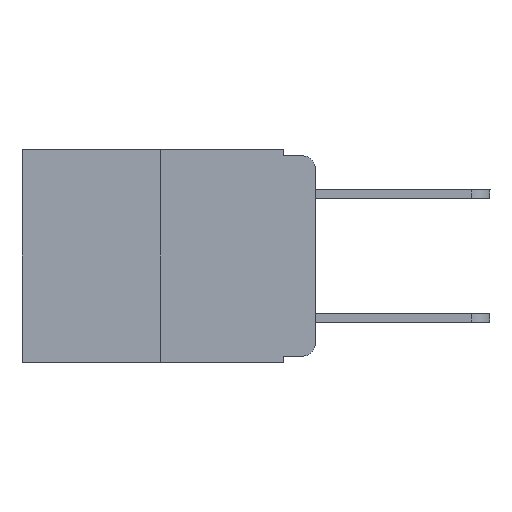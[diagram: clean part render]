
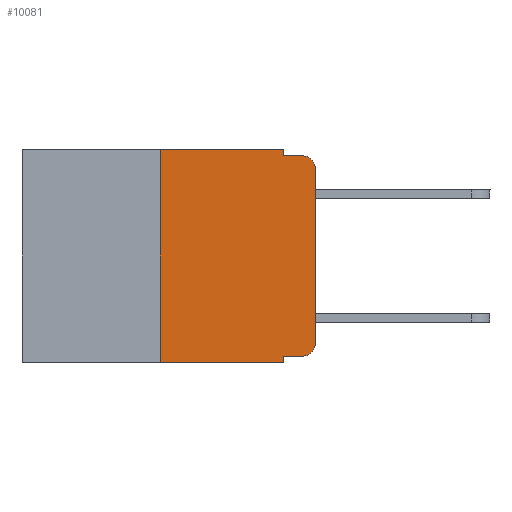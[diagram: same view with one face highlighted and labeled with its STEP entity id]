
A CAD part, left-side view. The second image highlights one B-rep face of the part: STEP entity #10081.
In plain terms, the highlighted planar face has unit normal (-1, 0, 0).
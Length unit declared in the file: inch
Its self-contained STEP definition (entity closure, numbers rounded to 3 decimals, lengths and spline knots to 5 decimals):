
#12 = LINE ( 'NONE', #4624, #12242 ) ;
#532 = LINE ( 'NONE', #13528, #14989 ) ;
#535 = CARTESIAN_POINT ( 'NONE',  ( 0., 0.473, 0. ) ) ;
#575 = LINE ( 'NONE', #5580, #6875 ) ;
#1215 = ORIENTED_EDGE ( 'NONE', *, *, #10044, .T. ) ;
#1301 = ORIENTED_EDGE ( 'NONE', *, *, #13924, .F. ) ;
#1306 = CARTESIAN_POINT ( 'NONE',  ( 0., 0.051, -0.333 ) ) ;
#1448 = VERTEX_POINT ( 'NONE', #2117 ) ;
#1495 = CARTESIAN_POINT ( 'NONE',  ( 0., 0., 0. ) ) ;
#1699 = AXIS2_PLACEMENT_3D ( 'NONE', #9700, #8440, #13099 ) ;
#1885 = VECTOR ( 'NONE', #6214, 39.37008 ) ;
#2117 = CARTESIAN_POINT ( 'NONE',  ( 0., 0.25, 0. ) ) ;
#2189 = CARTESIAN_POINT ( 'NONE',  ( 0., 0., -0.03 ) ) ;
#2199 = CARTESIAN_POINT ( 'NONE',  ( 0., 0.02, -0.03 ) ) ;
#2222 = AXIS2_PLACEMENT_3D ( 'NONE', #535, #2870, #3023 ) ;
#2604 = VERTEX_POINT ( 'NONE', #11430 ) ;
#2870 = DIRECTION ( 'NONE',  ( 1., 0., 0. ) ) ;
#3023 = DIRECTION ( 'NONE',  ( 0., 0., -1. ) ) ;
#3177 = VERTEX_POINT ( 'NONE', #2189 ) ;
#3796 = ORIENTED_EDGE ( 'NONE', *, *, #13596, .T. ) ;
#3999 = ORIENTED_EDGE ( 'NONE', *, *, #14926, .T. ) ;
#4545 = VERTEX_POINT ( 'NONE', #9415 ) ;
#4624 = CARTESIAN_POINT ( 'NONE',  ( 0., 0.051, -0.333 ) ) ;
#4720 = AXIS2_PLACEMENT_3D ( 'NONE', #2199, #6999, #8243 ) ;
#5358 = CARTESIAN_POINT ( 'NONE',  ( 0., 0., -0.313 ) ) ;
#5574 = EDGE_CURVE ( 'NONE', #10464, #13343, #575, .T. ) ;
#5580 = CARTESIAN_POINT ( 'NONE',  ( 0., 0.473, -0.343 ) ) ;
#5582 = EDGE_CURVE ( 'NONE', #1448, #9232, #6472, .T. ) ;
#5616 = EDGE_CURVE ( 'NONE', #10464, #1448, #7728, .T. ) ;
#5873 = VECTOR ( 'NONE', #10313, 39.37008 ) ;
#6121 = CARTESIAN_POINT ( 'NONE',  ( 0., 0.25, -0.343 ) ) ;
#6214 = DIRECTION ( 'NONE',  ( 0., 0., 1. ) ) ;
#6336 = PLANE ( 'NONE',  #2222 ) ;
#6472 = LINE ( 'NONE', #7798, #5873 ) ;
#6611 = DIRECTION ( 'NONE',  ( 0., -1., 0. ) ) ;
#6667 = VECTOR ( 'NONE', #11873, 39.37008 ) ;
#6875 = VECTOR ( 'NONE', #6611, 39.37008 ) ;
#6999 = DIRECTION ( 'NONE',  ( -1., 0., 0. ) ) ;
#7002 = DIRECTION ( 'NONE',  ( 0., -1., 0. ) ) ;
#7534 = EDGE_CURVE ( 'NONE', #4545, #10915, #532, .T. ) ;
#7728 = LINE ( 'NONE', #11512, #7870 ) ;
#7798 = CARTESIAN_POINT ( 'NONE',  ( 0., 0.473, 0. ) ) ;
#7870 = VECTOR ( 'NONE', #13725, 39.37008 ) ;
#8019 = VERTEX_POINT ( 'NONE', #5358 ) ;
#8243 = DIRECTION ( 'NONE',  ( 0., 0., -1. ) ) ;
#8440 = DIRECTION ( 'NONE',  ( -1., 0., 0. ) ) ;
#9109 = EDGE_CURVE ( 'NONE', #2604, #8019, #15269, .T. ) ;
#9232 = VERTEX_POINT ( 'NONE', #11213 ) ;
#9415 = CARTESIAN_POINT ( 'NONE',  ( 0., 0.051, -0.01 ) ) ;
#9454 = VECTOR ( 'NONE', #13312, 39.37008 ) ;
#9700 = CARTESIAN_POINT ( 'NONE',  ( 0., 0.02, -0.313 ) ) ;
#9874 = ORIENTED_EDGE ( 'NONE', *, *, #5574, .T. ) ;
#10044 = EDGE_CURVE ( 'NONE', #3177, #10915, #14299, .T. ) ;
#10081 = ADVANCED_FACE ( 'NONE', ( #13822 ), #6336, .F. ) ;
#10313 = DIRECTION ( 'NONE',  ( 0., -1., 0. ) ) ;
#10464 = VERTEX_POINT ( 'NONE', #6121 ) ;
#10856 = LINE ( 'NONE', #11890, #9454 ) ;
#10915 = VERTEX_POINT ( 'NONE', #13198 ) ;
#10997 = DIRECTION ( 'NONE',  ( 0., -1., 0. ) ) ;
#11213 = CARTESIAN_POINT ( 'NONE',  ( 0., 0.051, 0. ) ) ;
#11334 = LINE ( 'NONE', #1495, #1885 ) ;
#11430 = CARTESIAN_POINT ( 'NONE',  ( 0., 0.02, -0.333 ) ) ;
#11512 = CARTESIAN_POINT ( 'NONE',  ( 0., 0.25, 0. ) ) ;
#11873 = DIRECTION ( 'NONE',  ( 0., 0., -1. ) ) ;
#11890 = CARTESIAN_POINT ( 'NONE',  ( 0., 0.051, 0. ) ) ;
#12106 = CARTESIAN_POINT ( 'NONE',  ( 0., 0.051, 0. ) ) ;
#12242 = VECTOR ( 'NONE', #7002, 39.37008 ) ;
#13099 = DIRECTION ( 'NONE',  ( 0., 0., -1. ) ) ;
#13103 = ORIENTED_EDGE ( 'NONE', *, *, #14924, .F. ) ;
#13198 = CARTESIAN_POINT ( 'NONE',  ( 0., 0.02, -0.01 ) ) ;
#13312 = DIRECTION ( 'NONE',  ( 0., 0., -1. ) ) ;
#13343 = VERTEX_POINT ( 'NONE', #15279 ) ;
#13448 = ORIENTED_EDGE ( 'NONE', *, *, #5616, .F. ) ;
#13528 = CARTESIAN_POINT ( 'NONE',  ( 0., 0.051, -0.01 ) ) ;
#13596 = EDGE_CURVE ( 'NONE', #8019, #3177, #11334, .T. ) ;
#13725 = DIRECTION ( 'NONE',  ( 0., 0., 1. ) ) ;
#13822 = FACE_OUTER_BOUND ( 'NONE', #14544, .T. ) ;
#13924 = EDGE_CURVE ( 'NONE', #14674, #13343, #14542, .T. ) ;
#13982 = ORIENTED_EDGE ( 'NONE', *, *, #9109, .T. ) ;
#14299 = CIRCLE ( 'NONE', #4720, 0.02 ) ;
#14387 = ORIENTED_EDGE ( 'NONE', *, *, #5582, .F. ) ;
#14542 = LINE ( 'NONE', #12106, #6667 ) ;
#14544 = EDGE_LOOP ( 'NONE', ( #3796, #1215, #14838, #13103, #14387, #13448, #9874, #1301, #3999, #13982 ) ) ;
#14674 = VERTEX_POINT ( 'NONE', #1306 ) ;
#14838 = ORIENTED_EDGE ( 'NONE', *, *, #7534, .F. ) ;
#14924 = EDGE_CURVE ( 'NONE', #9232, #4545, #10856, .T. ) ;
#14926 = EDGE_CURVE ( 'NONE', #14674, #2604, #12, .T. ) ;
#14989 = VECTOR ( 'NONE', #10997, 39.37008 ) ;
#15269 = CIRCLE ( 'NONE', #1699, 0.02 ) ;
#15279 = CARTESIAN_POINT ( 'NONE',  ( 0., 0.051, -0.343 ) ) ;
